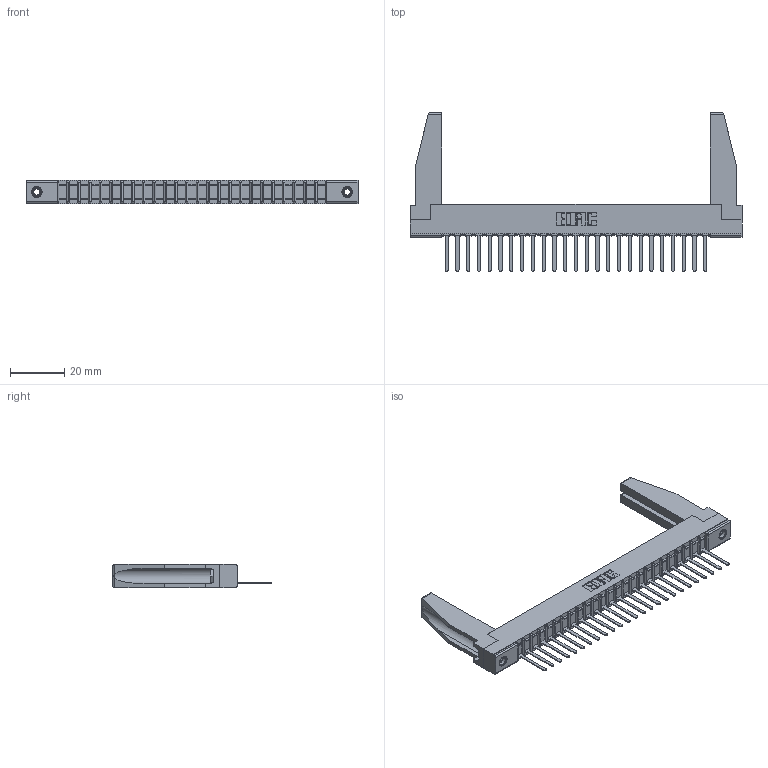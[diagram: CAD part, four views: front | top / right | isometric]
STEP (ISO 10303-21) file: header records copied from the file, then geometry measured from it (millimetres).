
FILE_DESCRIPTION (( 'STEP AP203' ), '1' );
FILE_NAME ('357-025-541-178.STEP', '2019-09-17T00:40:15', ( '' ), ( '' ), 'SwSTEP 2.0', 'SolidWorks 2016', '' );
FILE_SCHEMA (( 'CONFIG_CONTROL_DESIGN' ));
Length unit declared in the file: inch
Products named in the file (5): 357-025-541-178; 345-250-001_345-250-001-102; 307 Part_.156 Dia Mounting Holes; 307-290-002_541; 307-220-078
Assembly tree (30 placements, depth 2):
  357-025-541-178
    307 Part_.156 Dia Mounting Holes
    307-290-002_541  x25
    307-220-078  x2
    345-250-001_345-250-001-102  x2
Bounding box: 122.07 x 58.29 x 8.71 mm (x, y, z)
Volume: 12124.4 mm3; surface area: 19202.7 mm2
Topology: 30 solids, 30 shells, 2124 faces, 6453 edges, 4222 vertices
Faces by surface type: plane 1279, cylinder 777, sphere 52, cone 12, torus 4
Entity records: 26685 total; most frequent: CARTESIAN_POINT 4498, ORIENTED_EDGE 4444, DIRECTION 4334, EDGE_CURVE 2222, VECTOR 1698, LINE 1698, VERTEX_POINT 1440, AXIS2_PLACEMENT_3D 1318
